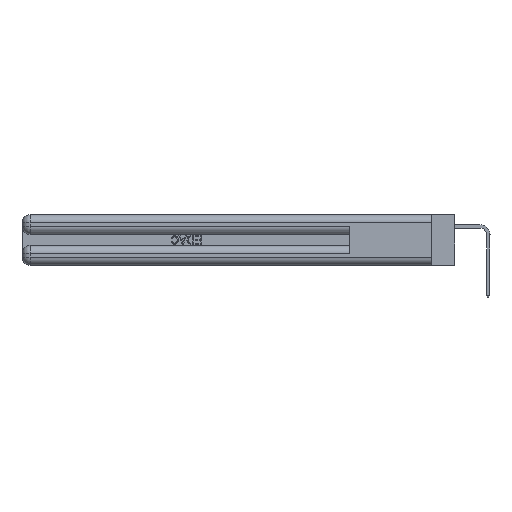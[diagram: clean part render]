
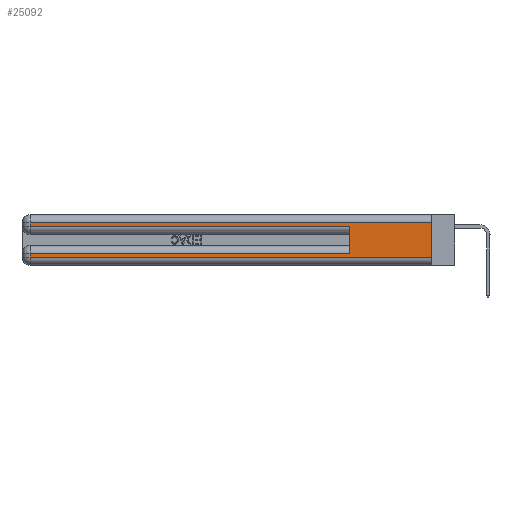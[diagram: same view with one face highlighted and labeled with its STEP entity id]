
A CAD part, left-side view. The second image highlights one B-rep face of the part: STEP entity #25092.
In plain terms, the highlighted planar face has unit normal (-1, 0, 0).
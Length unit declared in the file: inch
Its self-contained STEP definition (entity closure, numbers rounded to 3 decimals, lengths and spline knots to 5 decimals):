
#39 = EDGE_CURVE ( 'NONE', #39860, #12014, #15519, .T. ) ;
#461 = DIRECTION ( 'NONE',  ( 1., 0., 0. ) ) ;
#2394 = CARTESIAN_POINT ( 'NONE',  ( 0., 0., 0.37 ) ) ;
#2645 = LINE ( 'NONE', #36340, #9189 ) ;
#4082 = ORIENTED_EDGE ( 'NONE', *, *, #14093, .T. ) ;
#4630 = LINE ( 'NONE', #25279, #21782 ) ;
#5591 = ORIENTED_EDGE ( 'NONE', *, *, #22186, .T. ) ;
#5983 = DIRECTION ( 'NONE',  ( 0., 0., -1. ) ) ;
#7563 = DIRECTION ( 'NONE',  ( 0., 0., -1. ) ) ;
#8440 = VERTEX_POINT ( 'NONE', #19829 ) ;
#8839 = CARTESIAN_POINT ( 'NONE',  ( 0., 2.94, 0.285 ) ) ;
#8852 = VECTOR ( 'NONE', #32164, 39.37008 ) ;
#9189 = VECTOR ( 'NONE', #7563, 39.37008 ) ;
#9502 = CARTESIAN_POINT ( 'NONE',  ( 0., 0.6, 0.285 ) ) ;
#9556 = CARTESIAN_POINT ( 'NONE',  ( 0., 0., 0.06 ) ) ;
#9587 = ORIENTED_EDGE ( 'NONE', *, *, #36517, .F. ) ;
#9854 = LINE ( 'NONE', #35373, #8852 ) ;
#10027 = PLANE ( 'NONE',  #40679 ) ;
#11599 = EDGE_CURVE ( 'NONE', #20426, #26036, #2645, .T. ) ;
#11699 = VERTEX_POINT ( 'NONE', #20835 ) ;
#11821 = DIRECTION ( 'NONE',  ( 0., 1., 0. ) ) ;
#11935 = EDGE_CURVE ( 'NONE', #8440, #11966, #4630, .T. ) ;
#11962 = CARTESIAN_POINT ( 'NONE',  ( 0., 0.6, 0.145 ) ) ;
#11966 = VERTEX_POINT ( 'NONE', #34916 ) ;
#12014 = VERTEX_POINT ( 'NONE', #9502 ) ;
#12488 = CARTESIAN_POINT ( 'NONE',  ( 0., 0., 0.285 ) ) ;
#14093 = EDGE_CURVE ( 'NONE', #11699, #20426, #35343, .T. ) ;
#14458 = VERTEX_POINT ( 'NONE', #26552 ) ;
#15129 = VECTOR ( 'NONE', #41508, 39.37008 ) ;
#15204 = DIRECTION ( 'NONE',  ( 0., 0., 1. ) ) ;
#15519 = LINE ( 'NONE', #11962, #31605 ) ;
#15994 = EDGE_CURVE ( 'NONE', #11966, #14458, #22675, .T. ) ;
#16181 = ORIENTED_EDGE ( 'NONE', *, *, #11935, .T. ) ;
#16390 = CARTESIAN_POINT ( 'NONE',  ( 0., 0.6, 0.085 ) ) ;
#16527 = CARTESIAN_POINT ( 'NONE',  ( 0., 0., 0.37 ) ) ;
#16604 = EDGE_CURVE ( 'NONE', #26036, #12014, #35618, .T. ) ;
#19829 = CARTESIAN_POINT ( 'NONE',  ( 0., 2.94, 0.085 ) ) ;
#19916 = LINE ( 'NONE', #2394, #27423 ) ;
#20426 = VERTEX_POINT ( 'NONE', #27846 ) ;
#20835 = CARTESIAN_POINT ( 'NONE',  ( 0., 0., 0.31 ) ) ;
#21566 = CARTESIAN_POINT ( 'NONE',  ( 0., 0., 0.31 ) ) ;
#21756 = ORIENTED_EDGE ( 'NONE', *, *, #39, .F. ) ;
#21782 = VECTOR ( 'NONE', #5983, 39.37008 ) ;
#22186 = EDGE_CURVE ( 'NONE', #39860, #8440, #9854, .T. ) ;
#22675 = LINE ( 'NONE', #9556, #15129 ) ;
#23019 = DIRECTION ( 'NONE',  ( 0., 0., -1. ) ) ;
#25092 = ADVANCED_FACE ( 'NONE', ( #28354 ), #10027, .F. ) ;
#25279 = CARTESIAN_POINT ( 'NONE',  ( 0., 2.94, 0.37 ) ) ;
#25830 = VECTOR ( 'NONE', #11821, 39.37008 ) ;
#26036 = VERTEX_POINT ( 'NONE', #8839 ) ;
#26100 = EDGE_LOOP ( 'NONE', ( #9587, #4082, #39189, #28227, #21756, #5591, #16181, #33230 ) ) ;
#26552 = CARTESIAN_POINT ( 'NONE',  ( 0., 0., 0.06 ) ) ;
#27423 = VECTOR ( 'NONE', #34562, 39.37008 ) ;
#27846 = CARTESIAN_POINT ( 'NONE',  ( 0., 2.94, 0.31 ) ) ;
#28227 = ORIENTED_EDGE ( 'NONE', *, *, #16604, .T. ) ;
#28354 = FACE_OUTER_BOUND ( 'NONE', #26100, .T. ) ;
#31605 = VECTOR ( 'NONE', #15204, 39.37008 ) ;
#32164 = DIRECTION ( 'NONE',  ( 0., 1., 0. ) ) ;
#33230 = ORIENTED_EDGE ( 'NONE', *, *, #15994, .T. ) ;
#34562 = DIRECTION ( 'NONE',  ( 0., 0., -1. ) ) ;
#34625 = VECTOR ( 'NONE', #34930, 39.37008 ) ;
#34916 = CARTESIAN_POINT ( 'NONE',  ( 0., 2.94, 0.06 ) ) ;
#34930 = DIRECTION ( 'NONE',  ( 0., -1., 0. ) ) ;
#35343 = LINE ( 'NONE', #21566, #25830 ) ;
#35373 = CARTESIAN_POINT ( 'NONE',  ( 0., 0., 0.085 ) ) ;
#35618 = LINE ( 'NONE', #12488, #34625 ) ;
#36340 = CARTESIAN_POINT ( 'NONE',  ( 0., 2.94, 0.37 ) ) ;
#36517 = EDGE_CURVE ( 'NONE', #11699, #14458, #19916, .T. ) ;
#39189 = ORIENTED_EDGE ( 'NONE', *, *, #11599, .T. ) ;
#39860 = VERTEX_POINT ( 'NONE', #16390 ) ;
#40679 = AXIS2_PLACEMENT_3D ( 'NONE', #16527, #461, #23019 ) ;
#41508 = DIRECTION ( 'NONE',  ( 0., -1., 0. ) ) ;
